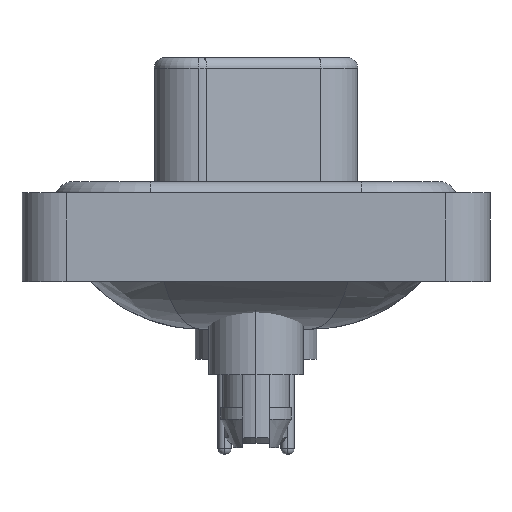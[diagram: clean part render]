
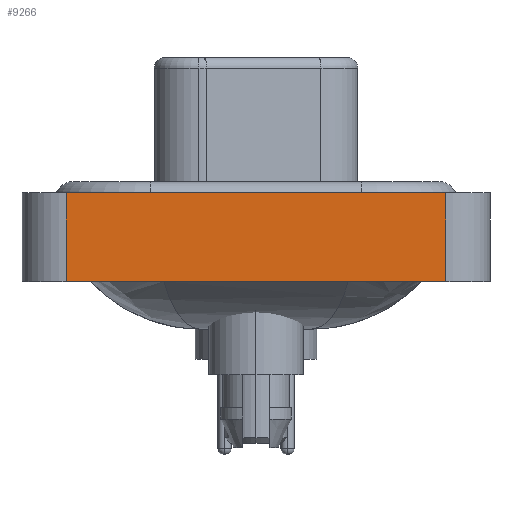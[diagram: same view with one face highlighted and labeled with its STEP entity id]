
A CAD part, left-side view. The second image highlights one B-rep face of the part: STEP entity #9266.
In plain terms, the highlighted planar face has unit normal (-1, 0, 0).
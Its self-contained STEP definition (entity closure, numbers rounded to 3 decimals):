
#820 = EDGE_CURVE ( 'NONE', #21455, #7008, #22639, .T. ) ;
#1356 = AXIS2_PLACEMENT_3D ( 'NONE', #12007, #2438, #19238 ) ;
#1945 = FACE_OUTER_BOUND ( 'NONE', #18185, .T. ) ;
#2438 = DIRECTION ( 'NONE',  ( -1., 0., 0. ) ) ;
#3107 = VECTOR ( 'NONE', #4712, 1000. ) ;
#4145 = CARTESIAN_POINT ( 'NONE',  ( -7.35, -8.55, 0.4 ) ) ;
#4712 = DIRECTION ( 'NONE',  ( 0., 0., 1. ) ) ;
#4768 = DIRECTION ( 'NONE',  ( 0., -1., 0. ) ) ;
#5656 = CARTESIAN_POINT ( 'NONE',  ( -7.35, 8.55, 0.4 ) ) ;
#5706 = EDGE_CURVE ( 'NONE', #9715, #21014, #6569, .T. ) ;
#6151 = EDGE_CURVE ( 'NONE', #21455, #9715, #23311, .T. ) ;
#6569 = LINE ( 'NONE', #22769, #15228 ) ;
#7008 = VERTEX_POINT ( 'NONE', #19055 ) ;
#7437 = VECTOR ( 'NONE', #14938, 1000. ) ;
#7801 = VECTOR ( 'NONE', #23266, 1000. ) ;
#9266 = ADVANCED_FACE ( 'NONE', ( #1945 ), #9326, .T. ) ;
#9326 = PLANE ( 'NONE',  #1356 ) ;
#9715 = VERTEX_POINT ( 'NONE', #5656 ) ;
#12007 = CARTESIAN_POINT ( 'NONE',  ( -7.35, -8.55, -3.6 ) ) ;
#14489 = LINE ( 'NONE', #16060, #7801 ) ;
#14938 = DIRECTION ( 'NONE',  ( 0., -1., 0. ) ) ;
#15228 = VECTOR ( 'NONE', #4768, 1000. ) ;
#15395 = ORIENTED_EDGE ( 'NONE', *, *, #5706, .F. ) ;
#16060 = CARTESIAN_POINT ( 'NONE',  ( -7.35, -8.55, -3.6 ) ) ;
#18185 = EDGE_LOOP ( 'NONE', ( #21034, #15395, #22716, #20544 ) ) ;
#18872 = EDGE_CURVE ( 'NONE', #7008, #21014, #14489, .T. ) ;
#19055 = CARTESIAN_POINT ( 'NONE',  ( -7.35, -8.55, -3.6 ) ) ;
#19238 = DIRECTION ( 'NONE',  ( 0., 0., 1. ) ) ;
#19431 = CARTESIAN_POINT ( 'NONE',  ( -7.35, 8.55, -3.6 ) ) ;
#20544 = ORIENTED_EDGE ( 'NONE', *, *, #820, .T. ) ;
#21014 = VERTEX_POINT ( 'NONE', #4145 ) ;
#21034 = ORIENTED_EDGE ( 'NONE', *, *, #18872, .T. ) ;
#21455 = VERTEX_POINT ( 'NONE', #19431 ) ;
#22394 = CARTESIAN_POINT ( 'NONE',  ( -7.35, -8.55, -3.6 ) ) ;
#22639 = LINE ( 'NONE', #22394, #7437 ) ;
#22716 = ORIENTED_EDGE ( 'NONE', *, *, #6151, .F. ) ;
#22769 = CARTESIAN_POINT ( 'NONE',  ( -7.35, -8.55, 0.4 ) ) ;
#23266 = DIRECTION ( 'NONE',  ( 0., 0., 1. ) ) ;
#23311 = LINE ( 'NONE', #23430, #3107 ) ;
#23430 = CARTESIAN_POINT ( 'NONE',  ( -7.35, 8.55, -3.6 ) ) ;
